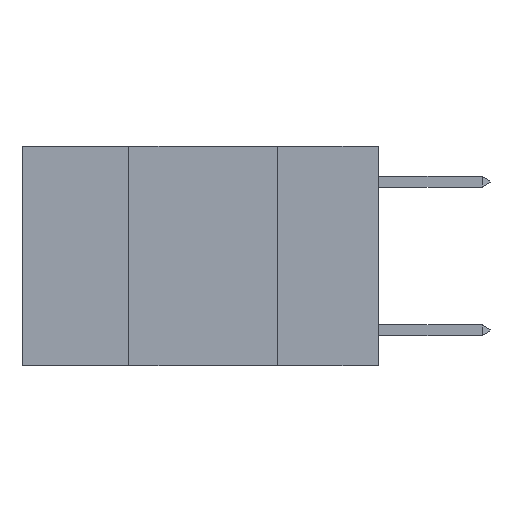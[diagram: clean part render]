
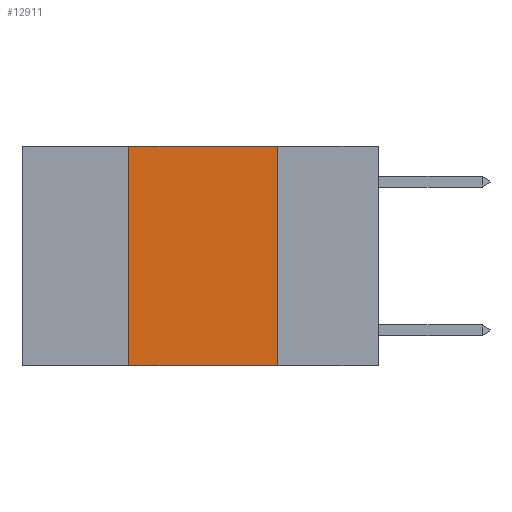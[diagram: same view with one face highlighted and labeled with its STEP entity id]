
A CAD part, left-side view. The second image highlights one B-rep face of the part: STEP entity #12911.
In plain terms, the highlighted planar face has unit normal (-1, 0, 0).
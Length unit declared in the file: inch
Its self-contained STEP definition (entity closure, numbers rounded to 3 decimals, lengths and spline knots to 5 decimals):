
#26 = LINE ( 'NONE', #13010, #10470 ) ;
#132 = EDGE_CURVE ( 'NONE', #12657, #1153, #7553, .T. ) ;
#540 = CARTESIAN_POINT ( 'NONE',  ( 0., 0.42, -0.37 ) ) ;
#1153 = VERTEX_POINT ( 'NONE', #14664 ) ;
#1236 = DIRECTION ( 'NONE',  ( 0., 0., -1. ) ) ;
#1430 = CARTESIAN_POINT ( 'NONE',  ( 0., 0.17, -0.37 ) ) ;
#2306 = DIRECTION ( 'NONE',  ( 0., -1., 0. ) ) ;
#2320 = ORIENTED_EDGE ( 'NONE', *, *, #132, .F. ) ;
#2642 = EDGE_CURVE ( 'NONE', #6889, #12657, #4463, .T. ) ;
#3263 = CARTESIAN_POINT ( 'NONE',  ( 0., 0.42, 0. ) ) ;
#3288 = ORIENTED_EDGE ( 'NONE', *, *, #16896, .T. ) ;
#4220 = DIRECTION ( 'NONE',  ( 1., 0., 0. ) ) ;
#4312 = CARTESIAN_POINT ( 'NONE',  ( 0., 0.6, 0. ) ) ;
#4463 = LINE ( 'NONE', #3263, #13869 ) ;
#5966 = ORIENTED_EDGE ( 'NONE', *, *, #10560, .F. ) ;
#6503 = ORIENTED_EDGE ( 'NONE', *, *, #2642, .F. ) ;
#6729 = VECTOR ( 'NONE', #12596, 39.37008 ) ;
#6889 = VERTEX_POINT ( 'NONE', #540 ) ;
#7347 = CARTESIAN_POINT ( 'NONE',  ( 0., 0.6, -0.37 ) ) ;
#7553 = LINE ( 'NONE', #8853, #15399 ) ;
#8853 = CARTESIAN_POINT ( 'NONE',  ( 0., 0.6, 0. ) ) ;
#9717 = DIRECTION ( 'NONE',  ( 0., 0., 1. ) ) ;
#10470 = VECTOR ( 'NONE', #1236, 39.37008 ) ;
#10560 = EDGE_CURVE ( 'NONE', #1153, #13646, #26, .T. ) ;
#10793 = EDGE_LOOP ( 'NONE', ( #5966, #2320, #6503, #3288 ) ) ;
#11689 = AXIS2_PLACEMENT_3D ( 'NONE', #4312, #4220, #12301 ) ;
#12301 = DIRECTION ( 'NONE',  ( 0., 0., -1. ) ) ;
#12569 = CARTESIAN_POINT ( 'NONE',  ( 0., 0.42, 0. ) ) ;
#12596 = DIRECTION ( 'NONE',  ( 0., -1., 0. ) ) ;
#12657 = VERTEX_POINT ( 'NONE', #12569 ) ;
#12751 = LINE ( 'NONE', #7347, #6729 ) ;
#12911 = ADVANCED_FACE ( 'NONE', ( #14769 ), #13407, .F. ) ;
#13010 = CARTESIAN_POINT ( 'NONE',  ( 0., 0.17, 0. ) ) ;
#13407 = PLANE ( 'NONE',  #11689 ) ;
#13646 = VERTEX_POINT ( 'NONE', #1430 ) ;
#13869 = VECTOR ( 'NONE', #9717, 39.37008 ) ;
#14664 = CARTESIAN_POINT ( 'NONE',  ( 0., 0.17, 0. ) ) ;
#14769 = FACE_OUTER_BOUND ( 'NONE', #10793, .T. ) ;
#15399 = VECTOR ( 'NONE', #2306, 39.37008 ) ;
#16896 = EDGE_CURVE ( 'NONE', #6889, #13646, #12751, .T. ) ;
